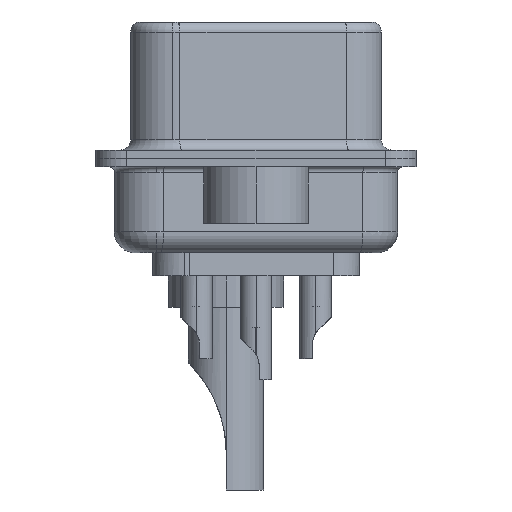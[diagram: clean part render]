
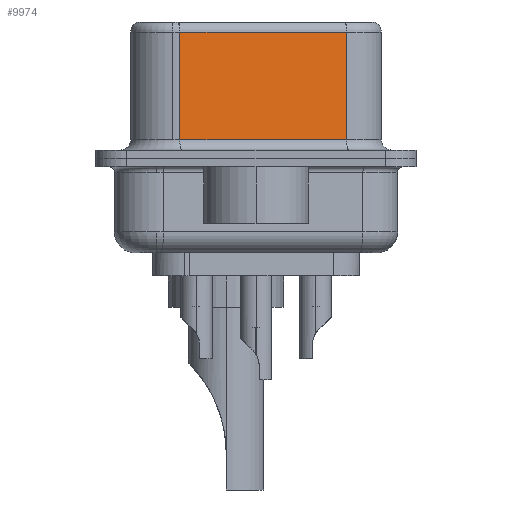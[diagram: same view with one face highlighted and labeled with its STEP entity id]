
A CAD part, left-side view. The second image highlights one B-rep face of the part: STEP entity #9974.
In plain terms, the highlighted planar face has unit normal (-0.985, -0.174, 0).
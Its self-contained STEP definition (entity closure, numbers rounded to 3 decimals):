
#594 = EDGE_LOOP ( 'NONE', ( #6146, #17769, #11828, #26575 ) ) ;
#827 = VERTEX_POINT ( 'NONE', #14072 ) ;
#2270 = CARTESIAN_POINT ( 'NONE',  ( 3.73, 3.628, 6.52 ) ) ;
#2543 = DIRECTION ( 'NONE',  ( -0.174, 0.985, 0. ) ) ;
#2592 = LINE ( 'NONE', #17451, #14156 ) ;
#2785 = DIRECTION ( 'NONE',  ( 0.174, -0.985, 0. ) ) ;
#3663 = DIRECTION ( 'NONE',  ( 0., 0., -1. ) ) ;
#4213 = VERTEX_POINT ( 'NONE', #15016 ) ;
#4514 = VECTOR ( 'NONE', #13477, 1000. ) ;
#4990 = EDGE_CURVE ( 'NONE', #5694, #827, #11120, .T. ) ;
#5694 = VERTEX_POINT ( 'NONE', #17361 ) ;
#6146 = ORIENTED_EDGE ( 'NONE', *, *, #12543, .F. ) ;
#6626 = DIRECTION ( 'NONE',  ( -0.174, 0.985, 0. ) ) ;
#9285 = DIRECTION ( 'NONE',  ( 0.985, 0.174, 0. ) ) ;
#9846 = VERTEX_POINT ( 'NONE', #11012 ) ;
#9974 = ADVANCED_FACE ( 'NONE', ( #14171 ), #20902, .F. ) ;
#10730 = AXIS2_PLACEMENT_3D ( 'NONE', #18592, #9285, #2543 ) ;
#11012 = CARTESIAN_POINT ( 'NONE',  ( 5.132, -4.322, 6.02 ) ) ;
#11120 = LINE ( 'NONE', #28073, #16569 ) ;
#11828 = ORIENTED_EDGE ( 'NONE', *, *, #17463, .T. ) ;
#12543 = EDGE_CURVE ( 'NONE', #9846, #827, #2592, .T. ) ;
#13075 = LINE ( 'NONE', #23091, #19935 ) ;
#13477 = DIRECTION ( 'NONE',  ( 0., 0., -1. ) ) ;
#14072 = CARTESIAN_POINT ( 'NONE',  ( 5.132, -4.322, 0.9 ) ) ;
#14156 = VECTOR ( 'NONE', #3663, 1000. ) ;
#14171 = FACE_OUTER_BOUND ( 'NONE', #594, .T. ) ;
#15016 = CARTESIAN_POINT ( 'NONE',  ( 3.73, 3.628, 6.02 ) ) ;
#15354 = LINE ( 'NONE', #2270, #4514 ) ;
#16569 = VECTOR ( 'NONE', #2785, 1000. ) ;
#17361 = CARTESIAN_POINT ( 'NONE',  ( 3.73, 3.628, 0.9 ) ) ;
#17451 = CARTESIAN_POINT ( 'NONE',  ( 5.132, -4.322, 6.52 ) ) ;
#17463 = EDGE_CURVE ( 'NONE', #4213, #5694, #15354, .T. ) ;
#17769 = ORIENTED_EDGE ( 'NONE', *, *, #26238, .T. ) ;
#18592 = CARTESIAN_POINT ( 'NONE',  ( 5.132, -4.322, 6.52 ) ) ;
#19935 = VECTOR ( 'NONE', #6626, 1000. ) ;
#20902 = PLANE ( 'NONE',  #10730 ) ;
#23091 = CARTESIAN_POINT ( 'NONE',  ( 5.132, -4.322, 6.02 ) ) ;
#26238 = EDGE_CURVE ( 'NONE', #9846, #4213, #13075, .T. ) ;
#26575 = ORIENTED_EDGE ( 'NONE', *, *, #4990, .T. ) ;
#28073 = CARTESIAN_POINT ( 'NONE',  ( 5.132, -4.322, 0.9 ) ) ;
